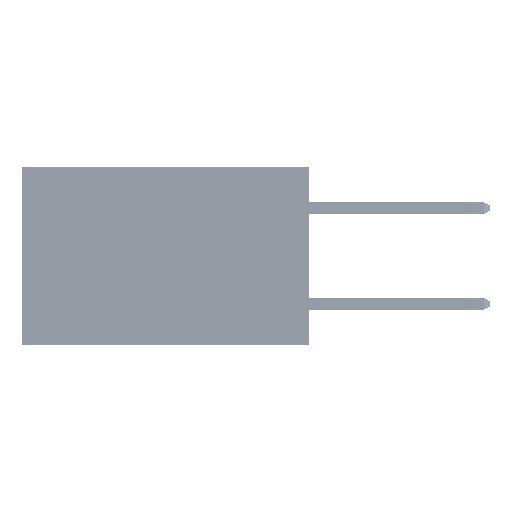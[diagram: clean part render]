
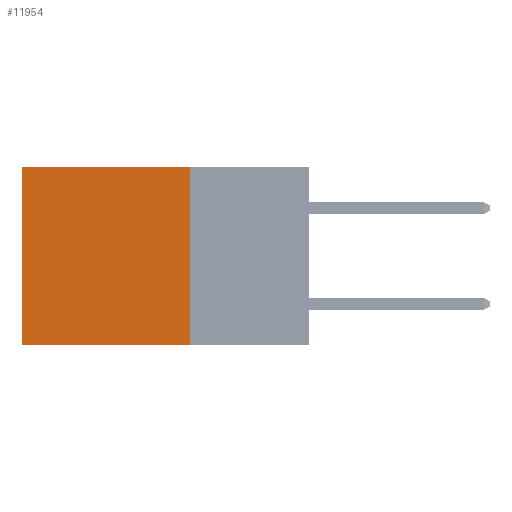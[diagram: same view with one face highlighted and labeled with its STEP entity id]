
A CAD part, left-side view. The second image highlights one B-rep face of the part: STEP entity #11954.
In plain terms, the highlighted planar face has unit normal (-1, 0, 0).
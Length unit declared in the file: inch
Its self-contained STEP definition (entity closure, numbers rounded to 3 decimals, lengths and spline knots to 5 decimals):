
#346 = DIRECTION ( 'NONE',  ( 0., 1., 0. ) ) ;
#498 = CARTESIAN_POINT ( 'NONE',  ( 0.2875, 0.25, 0. ) ) ;
#1120 = CARTESIAN_POINT ( 'NONE',  ( 0.2875, 0.25, 0. ) ) ;
#4129 = PLANE ( 'NONE',  #15911 ) ;
#4586 = VECTOR ( 'NONE', #28008, 39.37008 ) ;
#8616 = FACE_OUTER_BOUND ( 'NONE', #26614, .T. ) ;
#9850 = LINE ( 'NONE', #27853, #4586 ) ;
#11954 = ADVANCED_FACE ( 'NONE', ( #8616 ), #4129, .F. ) ;
#12061 = VERTEX_POINT ( 'NONE', #47205 ) ;
#12452 = CARTESIAN_POINT ( 'NONE',  ( 0.2875, 0.25, -0.37 ) ) ;
#13358 = CARTESIAN_POINT ( 'NONE',  ( 0.2875, 0.6, -0.37 ) ) ;
#15911 = AXIS2_PLACEMENT_3D ( 'NONE', #498, #42723, #27581 ) ;
#15916 = LINE ( 'NONE', #1120, #42883 ) ;
#16085 = CARTESIAN_POINT ( 'NONE',  ( 0.2875, 0.25, -0.37 ) ) ;
#17040 = CARTESIAN_POINT ( 'NONE',  ( 0.2875, 0.25, 0. ) ) ;
#21407 = VERTEX_POINT ( 'NONE', #17040 ) ;
#24516 = ORIENTED_EDGE ( 'NONE', *, *, #43696, .T. ) ;
#26614 = EDGE_LOOP ( 'NONE', ( #24516, #46835, #31222, #33483 ) ) ;
#27302 = LINE ( 'NONE', #32893, #33834 ) ;
#27581 = DIRECTION ( 'NONE',  ( 0., 0., -1. ) ) ;
#27853 = CARTESIAN_POINT ( 'NONE',  ( 0.2875, 0.25, 0. ) ) ;
#28008 = DIRECTION ( 'NONE',  ( 0., 0., -1. ) ) ;
#28050 = DIRECTION ( 'NONE',  ( 0., 1., 0. ) ) ;
#31222 = ORIENTED_EDGE ( 'NONE', *, *, #45163, .F. ) ;
#32893 = CARTESIAN_POINT ( 'NONE',  ( 0.2875, 0.6, 0. ) ) ;
#33483 = ORIENTED_EDGE ( 'NONE', *, *, #44213, .T. ) ;
#33834 = VECTOR ( 'NONE', #40709, 39.37008 ) ;
#35022 = EDGE_CURVE ( 'NONE', #43445, #36640, #40362, .T. ) ;
#36640 = VERTEX_POINT ( 'NONE', #13358 ) ;
#40362 = LINE ( 'NONE', #16085, #42782 ) ;
#40709 = DIRECTION ( 'NONE',  ( 0., 0., -1. ) ) ;
#42723 = DIRECTION ( 'NONE',  ( 1., 0., 0. ) ) ;
#42782 = VECTOR ( 'NONE', #346, 39.37008 ) ;
#42883 = VECTOR ( 'NONE', #28050, 39.37008 ) ;
#43445 = VERTEX_POINT ( 'NONE', #12452 ) ;
#43696 = EDGE_CURVE ( 'NONE', #12061, #36640, #27302, .T. ) ;
#44213 = EDGE_CURVE ( 'NONE', #21407, #12061, #15916, .T. ) ;
#45163 = EDGE_CURVE ( 'NONE', #21407, #43445, #9850, .T. ) ;
#46835 = ORIENTED_EDGE ( 'NONE', *, *, #35022, .F. ) ;
#47205 = CARTESIAN_POINT ( 'NONE',  ( 0.2875, 0.6, 0. ) ) ;
